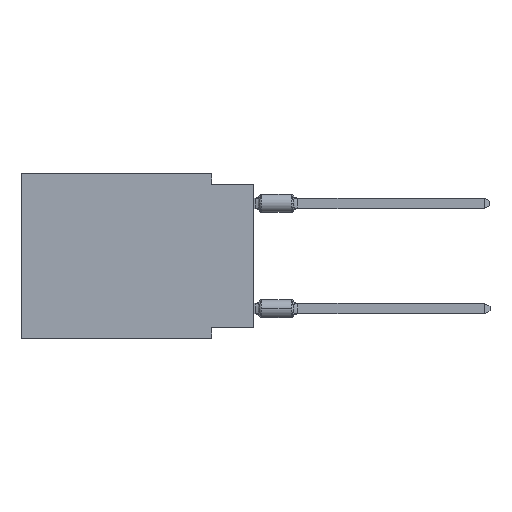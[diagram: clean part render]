
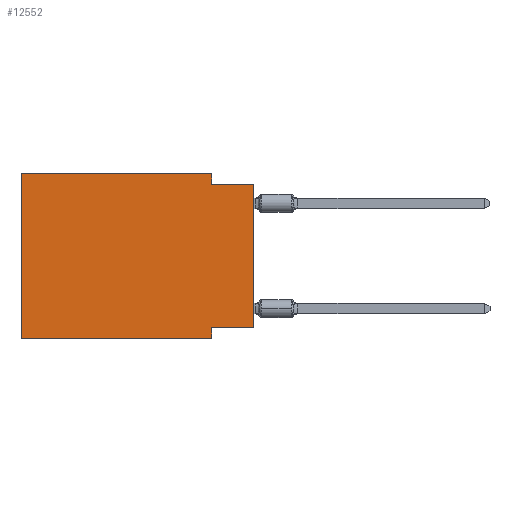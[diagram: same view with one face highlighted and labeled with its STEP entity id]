
A CAD part, left-side view. The second image highlights one B-rep face of the part: STEP entity #12552.
In plain terms, the highlighted planar face has unit normal (-1, 0, 0).
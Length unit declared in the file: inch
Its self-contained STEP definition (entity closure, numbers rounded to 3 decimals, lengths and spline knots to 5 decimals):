
#196 = DIRECTION ( 'NONE',  ( 0., -1., 0. ) ) ;
#520 = EDGE_CURVE ( 'NONE', #8857, #11531, #1817, .T. ) ;
#621 = CARTESIAN_POINT ( 'NONE',  ( 0., 0., 0. ) ) ;
#883 = DIRECTION ( 'NONE',  ( 0., 1., 0. ) ) ;
#1010 = CARTESIAN_POINT ( 'NONE',  ( 0., 0.1, -0.365 ) ) ;
#1047 = VECTOR ( 'NONE', #8323, 39.37008 ) ;
#1210 = LINE ( 'NONE', #6494, #15026 ) ;
#1402 = CARTESIAN_POINT ( 'NONE',  ( 0., 0.1, 0. ) ) ;
#1432 = EDGE_CURVE ( 'NONE', #3859, #10115, #8705, .T. ) ;
#1817 = LINE ( 'NONE', #1402, #1047 ) ;
#2029 = EDGE_CURVE ( 'NONE', #10115, #8857, #1210, .T. ) ;
#2118 = PLANE ( 'NONE',  #15479 ) ;
#2358 = CARTESIAN_POINT ( 'NONE',  ( 0., 0., -0.365 ) ) ;
#3159 = EDGE_CURVE ( 'NONE', #14667, #12364, #11401, .T. ) ;
#3351 = VECTOR ( 'NONE', #16257, 39.37008 ) ;
#3503 = CARTESIAN_POINT ( 'NONE',  ( 0., 0., -0.025 ) ) ;
#3624 = LINE ( 'NONE', #15705, #16848 ) ;
#3859 = VERTEX_POINT ( 'NONE', #13967 ) ;
#4709 = DIRECTION ( 'NONE',  ( 0., 0., 1. ) ) ;
#4911 = DIRECTION ( 'NONE',  ( 0., 0., -1. ) ) ;
#5810 = ORIENTED_EDGE ( 'NONE', *, *, #9048, .T. ) ;
#6009 = CARTESIAN_POINT ( 'NONE',  ( 0., 0.55, 0. ) ) ;
#6034 = EDGE_CURVE ( 'NONE', #14667, #6289, #12544, .T. ) ;
#6171 = DIRECTION ( 'NONE',  ( 0., -1., 0. ) ) ;
#6199 = ORIENTED_EDGE ( 'NONE', *, *, #1432, .F. ) ;
#6289 = VERTEX_POINT ( 'NONE', #12078 ) ;
#6494 = CARTESIAN_POINT ( 'NONE',  ( 0., 0.55, 0. ) ) ;
#7127 = VERTEX_POINT ( 'NONE', #15871 ) ;
#7411 = DIRECTION ( 'NONE',  ( 0., 0., -1. ) ) ;
#7458 = VECTOR ( 'NONE', #196, 39.37008 ) ;
#7597 = ORIENTED_EDGE ( 'NONE', *, *, #520, .F. ) ;
#8082 = CARTESIAN_POINT ( 'NONE',  ( 0., 0.1, -0.025 ) ) ;
#8259 = CARTESIAN_POINT ( 'NONE',  ( 0., 0.1, 0. ) ) ;
#8323 = DIRECTION ( 'NONE',  ( 0., 0., -1. ) ) ;
#8705 = LINE ( 'NONE', #6009, #13682 ) ;
#8720 = EDGE_LOOP ( 'NONE', ( #9263, #14736, #7597, #9576, #6199, #5810, #15068, #13283 ) ) ;
#8857 = VERTEX_POINT ( 'NONE', #8259 ) ;
#8883 = LINE ( 'NONE', #3503, #7458 ) ;
#9048 = EDGE_CURVE ( 'NONE', #3859, #7127, #12964, .T. ) ;
#9263 = ORIENTED_EDGE ( 'NONE', *, *, #6034, .T. ) ;
#9576 = ORIENTED_EDGE ( 'NONE', *, *, #2029, .F. ) ;
#10115 = VERTEX_POINT ( 'NONE', #13797 ) ;
#10360 = CARTESIAN_POINT ( 'NONE',  ( 0., 0., -0.365 ) ) ;
#10502 = DIRECTION ( 'NONE',  ( 0., -1., 0. ) ) ;
#11249 = CARTESIAN_POINT ( 'NONE',  ( 0., 0.55, 0. ) ) ;
#11401 = LINE ( 'NONE', #2358, #16230 ) ;
#11531 = VERTEX_POINT ( 'NONE', #8082 ) ;
#12078 = CARTESIAN_POINT ( 'NONE',  ( 0., 0., -0.025 ) ) ;
#12306 = EDGE_CURVE ( 'NONE', #12364, #7127, #3624, .T. ) ;
#12364 = VERTEX_POINT ( 'NONE', #1010 ) ;
#12544 = LINE ( 'NONE', #621, #3351 ) ;
#12552 = ADVANCED_FACE ( 'NONE', ( #16386 ), #2118, .F. ) ;
#12964 = LINE ( 'NONE', #15832, #16673 ) ;
#13283 = ORIENTED_EDGE ( 'NONE', *, *, #3159, .F. ) ;
#13682 = VECTOR ( 'NONE', #4709, 39.37008 ) ;
#13797 = CARTESIAN_POINT ( 'NONE',  ( 0., 0.55, 0. ) ) ;
#13967 = CARTESIAN_POINT ( 'NONE',  ( 0., 0.55, -0.39 ) ) ;
#14667 = VERTEX_POINT ( 'NONE', #10360 ) ;
#14736 = ORIENTED_EDGE ( 'NONE', *, *, #14763, .F. ) ;
#14763 = EDGE_CURVE ( 'NONE', #11531, #6289, #8883, .T. ) ;
#15026 = VECTOR ( 'NONE', #10502, 39.37008 ) ;
#15068 = ORIENTED_EDGE ( 'NONE', *, *, #12306, .F. ) ;
#15427 = DIRECTION ( 'NONE',  ( 1., 0., 0. ) ) ;
#15479 = AXIS2_PLACEMENT_3D ( 'NONE', #11249, #15427, #7411 ) ;
#15705 = CARTESIAN_POINT ( 'NONE',  ( 0., 0.1, -0.39 ) ) ;
#15832 = CARTESIAN_POINT ( 'NONE',  ( 0., 0.55, -0.39 ) ) ;
#15871 = CARTESIAN_POINT ( 'NONE',  ( 0., 0.1, -0.39 ) ) ;
#16230 = VECTOR ( 'NONE', #883, 39.37008 ) ;
#16257 = DIRECTION ( 'NONE',  ( 0., 0., 1. ) ) ;
#16386 = FACE_OUTER_BOUND ( 'NONE', #8720, .T. ) ;
#16673 = VECTOR ( 'NONE', #6171, 39.37008 ) ;
#16848 = VECTOR ( 'NONE', #4911, 39.37008 ) ;
